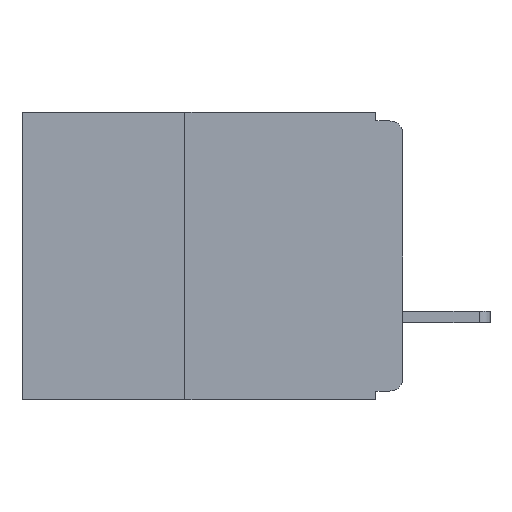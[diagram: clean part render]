
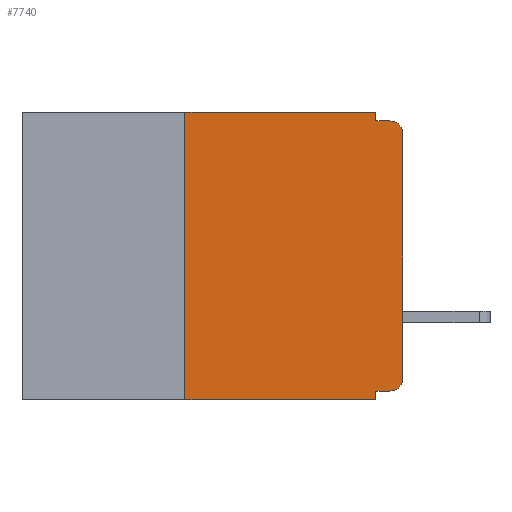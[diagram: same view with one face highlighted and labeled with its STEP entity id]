
A CAD part, left-side view. The second image highlights one B-rep face of the part: STEP entity #7740.
In plain terms, the highlighted planar face has unit normal (-1, 0, 0).
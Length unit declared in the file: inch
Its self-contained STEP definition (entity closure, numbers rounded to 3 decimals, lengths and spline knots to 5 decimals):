
#261 = AXIS2_PLACEMENT_3D ( 'NONE', #6675, #17638, #8265 ) ;
#366 = AXIS2_PLACEMENT_3D ( 'NONE', #5209, #2750, #19640 ) ;
#421 = VERTEX_POINT ( 'NONE', #9399 ) ;
#672 = CIRCLE ( 'NONE', #366, 0.015 ) ;
#741 = CIRCLE ( 'NONE', #261, 0.015 ) ;
#784 = DIRECTION ( 'NONE',  ( 0., -1., 0. ) ) ;
#793 = VERTEX_POINT ( 'NONE', #11429 ) ;
#938 = CARTESIAN_POINT ( 'NONE',  ( 0., 0.437, 0. ) ) ;
#1052 = ORIENTED_EDGE ( 'NONE', *, *, #13202, .F. ) ;
#2116 = ORIENTED_EDGE ( 'NONE', *, *, #14095, .T. ) ;
#2162 = VECTOR ( 'NONE', #17261, 39.37008 ) ;
#2344 = EDGE_CURVE ( 'NONE', #3047, #8664, #3594, .T. ) ;
#2654 = LINE ( 'NONE', #6792, #10207 ) ;
#2696 = LINE ( 'NONE', #16785, #14913 ) ;
#2726 = EDGE_CURVE ( 'NONE', #793, #3047, #672, .T. ) ;
#2745 = CARTESIAN_POINT ( 'NONE',  ( 0., 0.031, -0.33 ) ) ;
#2750 = DIRECTION ( 'NONE',  ( -1., 0., 0. ) ) ;
#2823 = EDGE_CURVE ( 'NONE', #4559, #12792, #11070, .T. ) ;
#2948 = ORIENTED_EDGE ( 'NONE', *, *, #2726, .T. ) ;
#3047 = VERTEX_POINT ( 'NONE', #4346 ) ;
#3573 = VECTOR ( 'NONE', #784, 39.37008 ) ;
#3594 = LINE ( 'NONE', #14200, #7348 ) ;
#4295 = CARTESIAN_POINT ( 'NONE',  ( 0., 0.031, 0. ) ) ;
#4346 = CARTESIAN_POINT ( 'NONE',  ( 0., 0., -0.305 ) ) ;
#4559 = VERTEX_POINT ( 'NONE', #9375 ) ;
#4855 = EDGE_CURVE ( 'NONE', #793, #7681, #11712, .T. ) ;
#5209 = CARTESIAN_POINT ( 'NONE',  ( 0., 0.015, -0.305 ) ) ;
#5266 = VERTEX_POINT ( 'NONE', #6580 ) ;
#5949 = ORIENTED_EDGE ( 'NONE', *, *, #15293, .T. ) ;
#6212 = ORIENTED_EDGE ( 'NONE', *, *, #2823, .F. ) ;
#6277 = EDGE_CURVE ( 'NONE', #421, #4559, #16317, .T. ) ;
#6451 = ORIENTED_EDGE ( 'NONE', *, *, #14375, .F. ) ;
#6580 = CARTESIAN_POINT ( 'NONE',  ( 0., 0.015, -0.01 ) ) ;
#6675 = CARTESIAN_POINT ( 'NONE',  ( 0., 0.015, -0.025 ) ) ;
#6792 = CARTESIAN_POINT ( 'NONE',  ( 0., 0.437, -0.33 ) ) ;
#7348 = VECTOR ( 'NONE', #11814, 39.37008 ) ;
#7681 = VERTEX_POINT ( 'NONE', #12817 ) ;
#7740 = ADVANCED_FACE ( 'NONE', ( #9656 ), #10263, .F. ) ;
#8169 = ORIENTED_EDGE ( 'NONE', *, *, #6277, .F. ) ;
#8265 = DIRECTION ( 'NONE',  ( 0., 0., -1. ) ) ;
#8381 = DIRECTION ( 'NONE',  ( 0., -1., 0. ) ) ;
#8664 = VERTEX_POINT ( 'NONE', #10489 ) ;
#8978 = DIRECTION ( 'NONE',  ( 0., -1., 0. ) ) ;
#9375 = CARTESIAN_POINT ( 'NONE',  ( 0., 0.25, 0. ) ) ;
#9399 = CARTESIAN_POINT ( 'NONE',  ( 0., 0.25, -0.33 ) ) ;
#9656 = FACE_OUTER_BOUND ( 'NONE', #20124, .T. ) ;
#10207 = VECTOR ( 'NONE', #8381, 39.37008 ) ;
#10263 = PLANE ( 'NONE',  #20277 ) ;
#10281 = DIRECTION ( 'NONE',  ( 0., 0., -1. ) ) ;
#10445 = DIRECTION ( 'NONE',  ( 1., 0., 0. ) ) ;
#10489 = CARTESIAN_POINT ( 'NONE',  ( 0., 0., -0.025 ) ) ;
#10557 = CARTESIAN_POINT ( 'NONE',  ( 0., 0.437, 0. ) ) ;
#11070 = LINE ( 'NONE', #938, #3573 ) ;
#11423 = VECTOR ( 'NONE', #18339, 39.37008 ) ;
#11429 = CARTESIAN_POINT ( 'NONE',  ( 0., 0.015, -0.32 ) ) ;
#11447 = ORIENTED_EDGE ( 'NONE', *, *, #4855, .F. ) ;
#11712 = LINE ( 'NONE', #13005, #2162 ) ;
#11814 = DIRECTION ( 'NONE',  ( 0., 0., 1. ) ) ;
#11982 = CARTESIAN_POINT ( 'NONE',  ( 0., 0.031, -0.01 ) ) ;
#12009 = CARTESIAN_POINT ( 'NONE',  ( 0., 0.031, -0.33 ) ) ;
#12182 = VECTOR ( 'NONE', #12636, 39.37008 ) ;
#12593 = CARTESIAN_POINT ( 'NONE',  ( 0., 0.25, -0.33 ) ) ;
#12636 = DIRECTION ( 'NONE',  ( 0., 0., 1. ) ) ;
#12792 = VERTEX_POINT ( 'NONE', #15180 ) ;
#12817 = CARTESIAN_POINT ( 'NONE',  ( 0., 0.031, -0.32 ) ) ;
#12850 = LINE ( 'NONE', #12009, #16491 ) ;
#13005 = CARTESIAN_POINT ( 'NONE',  ( 0., 0., -0.32 ) ) ;
#13202 = EDGE_CURVE ( 'NONE', #20370, #5266, #2696, .T. ) ;
#13601 = DIRECTION ( 'NONE',  ( 0., 0., -1. ) ) ;
#14095 = EDGE_CURVE ( 'NONE', #421, #14473, #2654, .T. ) ;
#14200 = CARTESIAN_POINT ( 'NONE',  ( 0., 0., 0. ) ) ;
#14375 = EDGE_CURVE ( 'NONE', #12792, #20370, #20173, .T. ) ;
#14473 = VERTEX_POINT ( 'NONE', #2745 ) ;
#14913 = VECTOR ( 'NONE', #8978, 39.37008 ) ;
#15180 = CARTESIAN_POINT ( 'NONE',  ( 0., 0.031, 0. ) ) ;
#15293 = EDGE_CURVE ( 'NONE', #8664, #5266, #741, .T. ) ;
#15530 = EDGE_CURVE ( 'NONE', #7681, #14473, #12850, .T. ) ;
#16317 = LINE ( 'NONE', #12593, #12182 ) ;
#16491 = VECTOR ( 'NONE', #13601, 39.37008 ) ;
#16785 = CARTESIAN_POINT ( 'NONE',  ( 0., 0., -0.01 ) ) ;
#17009 = ORIENTED_EDGE ( 'NONE', *, *, #15530, .F. ) ;
#17261 = DIRECTION ( 'NONE',  ( 0., 1., 0. ) ) ;
#17638 = DIRECTION ( 'NONE',  ( -1., 0., 0. ) ) ;
#18339 = DIRECTION ( 'NONE',  ( 0., 0., -1. ) ) ;
#19477 = ORIENTED_EDGE ( 'NONE', *, *, #2344, .T. ) ;
#19640 = DIRECTION ( 'NONE',  ( 0., 0., -1. ) ) ;
#20124 = EDGE_LOOP ( 'NONE', ( #19477, #5949, #1052, #6451, #6212, #8169, #2116, #17009, #11447, #2948 ) ) ;
#20173 = LINE ( 'NONE', #4295, #11423 ) ;
#20277 = AXIS2_PLACEMENT_3D ( 'NONE', #10557, #10445, #10281 ) ;
#20370 = VERTEX_POINT ( 'NONE', #11982 ) ;
